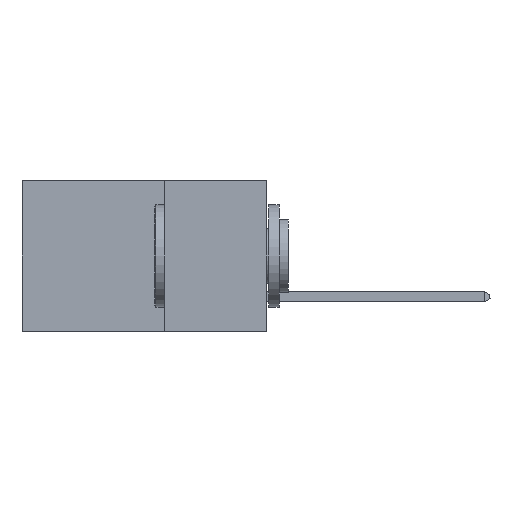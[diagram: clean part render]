
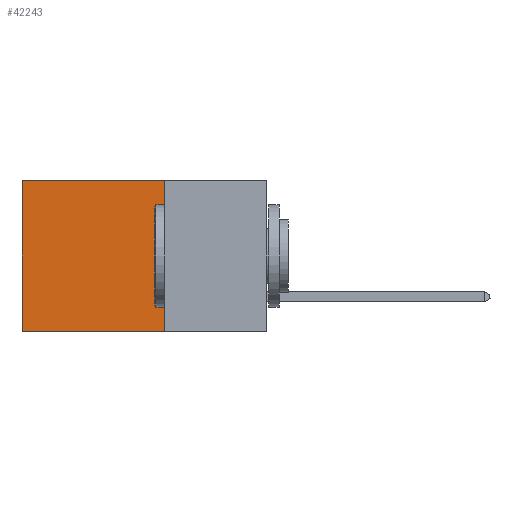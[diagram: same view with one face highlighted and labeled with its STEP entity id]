
A CAD part, left-side view. The second image highlights one B-rep face of the part: STEP entity #42243.
In plain terms, the highlighted planar face has unit normal (-1, 0, 0).
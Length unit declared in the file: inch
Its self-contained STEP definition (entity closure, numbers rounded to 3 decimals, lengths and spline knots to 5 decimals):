
#647 = ORIENTED_EDGE ( 'NONE', *, *, #23616, .T. ) ;
#1846 = VERTEX_POINT ( 'NONE', #8240 ) ;
#4589 = VECTOR ( 'NONE', #42887, 39.37008 ) ;
#7592 = ORIENTED_EDGE ( 'NONE', *, *, #10450, .T. ) ;
#7632 = VECTOR ( 'NONE', #17342, 39.37008 ) ;
#8240 = CARTESIAN_POINT ( 'NONE',  ( 0.2875, 0.6, 0. ) ) ;
#9956 = VERTEX_POINT ( 'NONE', #35447 ) ;
#10450 = EDGE_CURVE ( 'NONE', #1846, #40848, #28446, .T. ) ;
#11458 = EDGE_CURVE ( 'NONE', #33265, #9956, #27110, .T. ) ;
#11494 = ORIENTED_EDGE ( 'NONE', *, *, #28970, .F. ) ;
#13476 = CARTESIAN_POINT ( 'NONE',  ( 0.2875, 0.6, 0. ) ) ;
#13679 = CARTESIAN_POINT ( 'NONE',  ( 0.2875, 0.25, -0.37 ) ) ;
#13729 = DIRECTION ( 'NONE',  ( 1., 0., 0. ) ) ;
#17342 = DIRECTION ( 'NONE',  ( 0., 0., -1. ) ) ;
#18573 = CARTESIAN_POINT ( 'NONE',  ( 0.2875, 0.25, 0. ) ) ;
#18898 = CARTESIAN_POINT ( 'NONE',  ( 0.2875, 0.6, -0.37 ) ) ;
#20843 = VECTOR ( 'NONE', #33231, 39.37008 ) ;
#23616 = EDGE_CURVE ( 'NONE', #33265, #1846, #30539, .T. ) ;
#24897 = VECTOR ( 'NONE', #42699, 39.37008 ) ;
#27110 = LINE ( 'NONE', #38998, #24897 ) ;
#27240 = AXIS2_PLACEMENT_3D ( 'NONE', #35845, #13729, #39559 ) ;
#28227 = CARTESIAN_POINT ( 'NONE',  ( 0.2875, 0.25, 0. ) ) ;
#28446 = LINE ( 'NONE', #13476, #7632 ) ;
#28970 = EDGE_CURVE ( 'NONE', #9956, #40848, #34006, .T. ) ;
#30539 = LINE ( 'NONE', #18573, #20843 ) ;
#32085 = PLANE ( 'NONE',  #27240 ) ;
#33231 = DIRECTION ( 'NONE',  ( 0., 1., 0. ) ) ;
#33265 = VERTEX_POINT ( 'NONE', #28227 ) ;
#34006 = LINE ( 'NONE', #13679, #4589 ) ;
#35447 = CARTESIAN_POINT ( 'NONE',  ( 0.2875, 0.25, -0.37 ) ) ;
#35845 = CARTESIAN_POINT ( 'NONE',  ( 0.2875, 0.25, 0. ) ) ;
#38998 = CARTESIAN_POINT ( 'NONE',  ( 0.2875, 0.25, 0. ) ) ;
#39559 = DIRECTION ( 'NONE',  ( 0., 0., -1. ) ) ;
#40777 = EDGE_LOOP ( 'NONE', ( #7592, #11494, #41459, #647 ) ) ;
#40848 = VERTEX_POINT ( 'NONE', #18898 ) ;
#41459 = ORIENTED_EDGE ( 'NONE', *, *, #11458, .F. ) ;
#42243 = ADVANCED_FACE ( 'NONE', ( #43724 ), #32085, .F. ) ;
#42699 = DIRECTION ( 'NONE',  ( 0., 0., -1. ) ) ;
#42887 = DIRECTION ( 'NONE',  ( 0., 1., 0. ) ) ;
#43724 = FACE_OUTER_BOUND ( 'NONE', #40777, .T. ) ;
